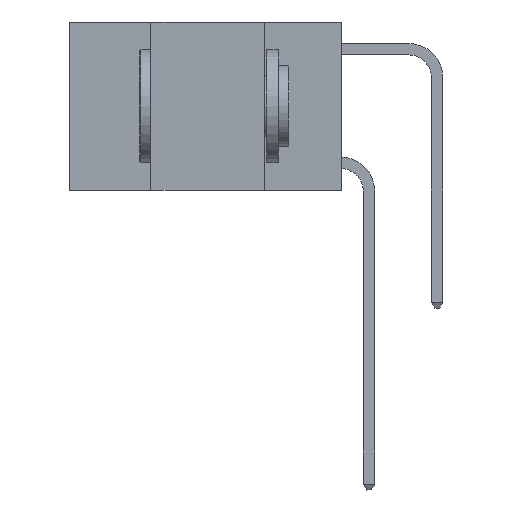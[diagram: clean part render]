
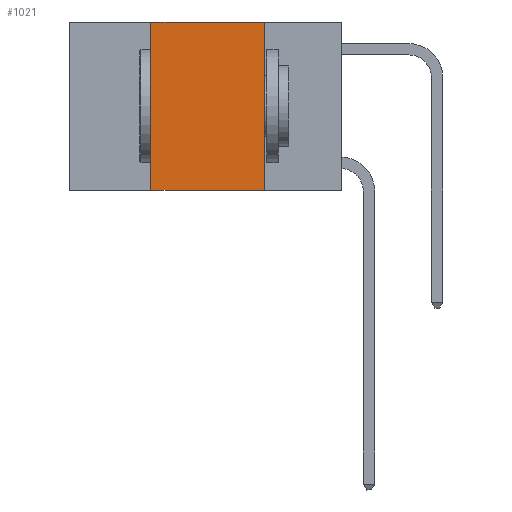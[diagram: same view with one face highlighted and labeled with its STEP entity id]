
A CAD part, left-side view. The second image highlights one B-rep face of the part: STEP entity #1021.
In plain terms, the highlighted planar face has unit normal (-1, 0, 0).
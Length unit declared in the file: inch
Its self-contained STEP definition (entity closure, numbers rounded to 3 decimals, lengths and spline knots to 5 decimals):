
#243 = PLANE ( 'NONE',  #18825 ) ;
#508 = CARTESIAN_POINT ( 'NONE',  ( 0., 0.6, 0. ) ) ;
#714 = VECTOR ( 'NONE', #10740, 39.37008 ) ;
#811 = LINE ( 'NONE', #3441, #23171 ) ;
#1021 = ADVANCED_FACE ( 'NONE', ( #24580 ), #243, .F. ) ;
#1455 = LINE ( 'NONE', #12875, #714 ) ;
#3441 = CARTESIAN_POINT ( 'NONE',  ( 0., 0.6, -0.37 ) ) ;
#4517 = ORIENTED_EDGE ( 'NONE', *, *, #24761, .F. ) ;
#4874 = ORIENTED_EDGE ( 'NONE', *, *, #8230, .F. ) ;
#5974 = LINE ( 'NONE', #18889, #10340 ) ;
#6735 = ORIENTED_EDGE ( 'NONE', *, *, #24343, .F. ) ;
#7213 = CARTESIAN_POINT ( 'NONE',  ( 0., 0.42, 0. ) ) ;
#7253 = DIRECTION ( 'NONE',  ( 0., -1., 0. ) ) ;
#7961 = EDGE_LOOP ( 'NONE', ( #4874, #4517, #6735, #27343 ) ) ;
#8230 = EDGE_CURVE ( 'NONE', #27719, #24194, #1455, .T. ) ;
#8500 = VERTEX_POINT ( 'NONE', #19876 ) ;
#10340 = VECTOR ( 'NONE', #23130, 39.37008 ) ;
#10740 = DIRECTION ( 'NONE',  ( 0., 0., -1. ) ) ;
#11214 = DIRECTION ( 'NONE',  ( 1., 0., 0. ) ) ;
#11666 = LINE ( 'NONE', #24204, #16617 ) ;
#12875 = CARTESIAN_POINT ( 'NONE',  ( 0., 0.17, 0. ) ) ;
#13028 = EDGE_CURVE ( 'NONE', #8500, #24194, #811, .T. ) ;
#16617 = VECTOR ( 'NONE', #7253, 39.37008 ) ;
#17401 = VERTEX_POINT ( 'NONE', #7213 ) ;
#18520 = DIRECTION ( 'NONE',  ( 0., -1., 0. ) ) ;
#18825 = AXIS2_PLACEMENT_3D ( 'NONE', #508, #11214, #19373 ) ;
#18889 = CARTESIAN_POINT ( 'NONE',  ( 0., 0.42, 0. ) ) ;
#19373 = DIRECTION ( 'NONE',  ( 0., 0., -1. ) ) ;
#19876 = CARTESIAN_POINT ( 'NONE',  ( 0., 0.42, -0.37 ) ) ;
#22673 = CARTESIAN_POINT ( 'NONE',  ( 0., 0.17, 0. ) ) ;
#22771 = CARTESIAN_POINT ( 'NONE',  ( 0., 0.17, -0.37 ) ) ;
#23130 = DIRECTION ( 'NONE',  ( 0., 0., 1. ) ) ;
#23171 = VECTOR ( 'NONE', #18520, 39.37008 ) ;
#24194 = VERTEX_POINT ( 'NONE', #22771 ) ;
#24204 = CARTESIAN_POINT ( 'NONE',  ( 0., 0.6, 0. ) ) ;
#24343 = EDGE_CURVE ( 'NONE', #8500, #17401, #5974, .T. ) ;
#24580 = FACE_OUTER_BOUND ( 'NONE', #7961, .T. ) ;
#24761 = EDGE_CURVE ( 'NONE', #17401, #27719, #11666, .T. ) ;
#27343 = ORIENTED_EDGE ( 'NONE', *, *, #13028, .T. ) ;
#27719 = VERTEX_POINT ( 'NONE', #22673 ) ;
